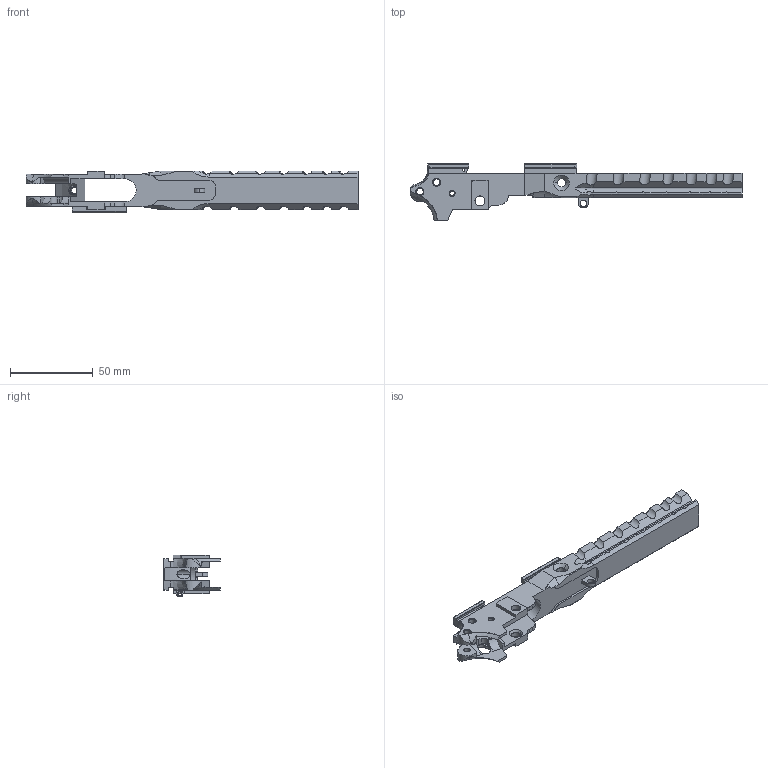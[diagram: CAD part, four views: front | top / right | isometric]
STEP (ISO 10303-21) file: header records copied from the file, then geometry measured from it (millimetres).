
FILE_DESCRIPTION (( 'STEP AP214' ), '1' );
FILE_NAME ('Frame_Single_Tactical_5Zoll.STEP', '2013-07-30T15:12:07', ( 'Asher' ), ( '' ), 'SwSTEP 2.0', 'SolidWorks 2013', '' );
FILE_SCHEMA (( 'AUTOMOTIVE_DESIGN' ));
Length unit declared in the file: millimetre
Products named in the file (1): Frame_Single_Tactical_5Zoll
Bounding box: 200.55 x 33.91 x 25.37 mm (x, y, z)
Volume: 31455.6 mm3; surface area: 22663.9 mm2
Topology: 1 solids, 1 shells, 321 faces, 922 edges, 602 vertices
Faces by surface type: plane 142, cylinder 126, cone 34, bspline 12, torus 7
Entity records: 11344 total; most frequent: CARTESIAN_POINT 3089, ORIENTED_EDGE 1844, DIRECTION 1598, EDGE_CURVE 922, VERTEX_POINT 602, AXIS2_PLACEMENT_3D 533, LINE 532, VECTOR 532
